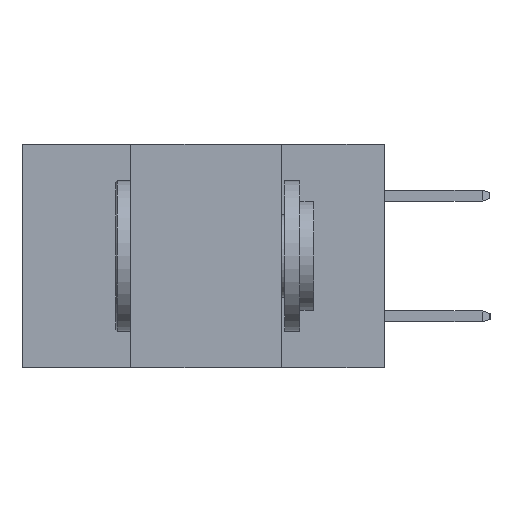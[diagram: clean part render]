
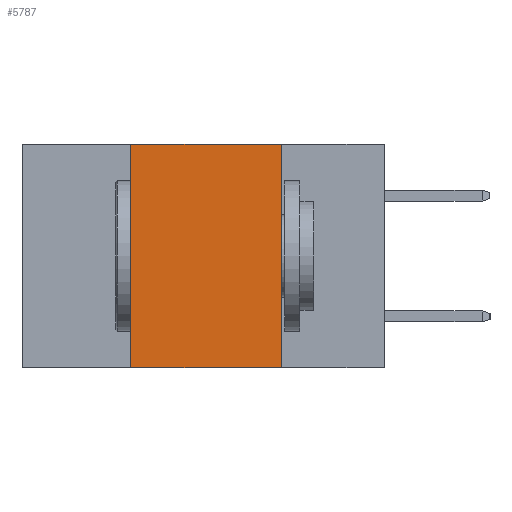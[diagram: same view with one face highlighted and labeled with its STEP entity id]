
A CAD part, left-side view. The second image highlights one B-rep face of the part: STEP entity #5787.
In plain terms, the highlighted planar face has unit normal (-1, 0, 0).
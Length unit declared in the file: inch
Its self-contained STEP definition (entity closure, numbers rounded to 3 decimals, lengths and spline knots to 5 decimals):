
#798 = DIRECTION ( 'NONE',  ( 0., -1., 0. ) ) ;
#810 = LINE ( 'NONE', #906, #7872 ) ;
#906 = CARTESIAN_POINT ( 'NONE',  ( 0., 0.6, -0.37 ) ) ;
#1136 = AXIS2_PLACEMENT_3D ( 'NONE', #13546, #12724, #12698 ) ;
#1267 = DIRECTION ( 'NONE',  ( 0., 0., -1. ) ) ;
#1579 = CARTESIAN_POINT ( 'NONE',  ( 0., 0.42, 0. ) ) ;
#3731 = EDGE_CURVE ( 'NONE', #10410, #9526, #810, .T. ) ;
#4265 = DIRECTION ( 'NONE',  ( 0., 0., 1. ) ) ;
#4597 = VECTOR ( 'NONE', #4265, 39.37008 ) ;
#4703 = CARTESIAN_POINT ( 'NONE',  ( 0., 0.42, -0.37 ) ) ;
#4722 = VECTOR ( 'NONE', #1267, 39.37008 ) ;
#5787 = ADVANCED_FACE ( 'NONE', ( #5931 ), #13348, .F. ) ;
#5931 = FACE_OUTER_BOUND ( 'NONE', #9434, .T. ) ;
#6168 = EDGE_CURVE ( 'NONE', #10410, #6540, #15103, .T. ) ;
#6540 = VERTEX_POINT ( 'NONE', #1579 ) ;
#7109 = ORIENTED_EDGE ( 'NONE', *, *, #3731, .T. ) ;
#7194 = CARTESIAN_POINT ( 'NONE',  ( 0., 0.6, 0. ) ) ;
#7720 = VERTEX_POINT ( 'NONE', #10384 ) ;
#7872 = VECTOR ( 'NONE', #798, 39.37008 ) ;
#8642 = LINE ( 'NONE', #17073, #4722 ) ;
#9151 = EDGE_CURVE ( 'NONE', #7720, #9526, #8642, .T. ) ;
#9434 = EDGE_LOOP ( 'NONE', ( #13053, #11210, #13285, #7109 ) ) ;
#9506 = CARTESIAN_POINT ( 'NONE',  ( 0., 0.17, -0.37 ) ) ;
#9526 = VERTEX_POINT ( 'NONE', #9506 ) ;
#9701 = EDGE_CURVE ( 'NONE', #6540, #7720, #14381, .T. ) ;
#9879 = CARTESIAN_POINT ( 'NONE',  ( 0., 0.42, -0.37 ) ) ;
#10384 = CARTESIAN_POINT ( 'NONE',  ( 0., 0.17, 0. ) ) ;
#10410 = VERTEX_POINT ( 'NONE', #9879 ) ;
#11210 = ORIENTED_EDGE ( 'NONE', *, *, #9701, .F. ) ;
#12698 = DIRECTION ( 'NONE',  ( 0., 0., -1. ) ) ;
#12724 = DIRECTION ( 'NONE',  ( 1., 0., 0. ) ) ;
#13053 = ORIENTED_EDGE ( 'NONE', *, *, #9151, .F. ) ;
#13285 = ORIENTED_EDGE ( 'NONE', *, *, #6168, .F. ) ;
#13348 = PLANE ( 'NONE',  #1136 ) ;
#13546 = CARTESIAN_POINT ( 'NONE',  ( 0., 0.6, 0. ) ) ;
#13551 = VECTOR ( 'NONE', #15064, 39.37008 ) ;
#14381 = LINE ( 'NONE', #7194, #13551 ) ;
#15064 = DIRECTION ( 'NONE',  ( 0., -1., 0. ) ) ;
#15103 = LINE ( 'NONE', #4703, #4597 ) ;
#17073 = CARTESIAN_POINT ( 'NONE',  ( 0., 0.17, -0.37 ) ) ;
